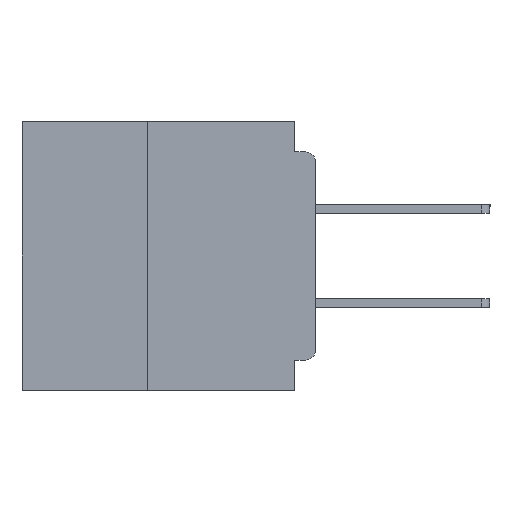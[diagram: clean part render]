
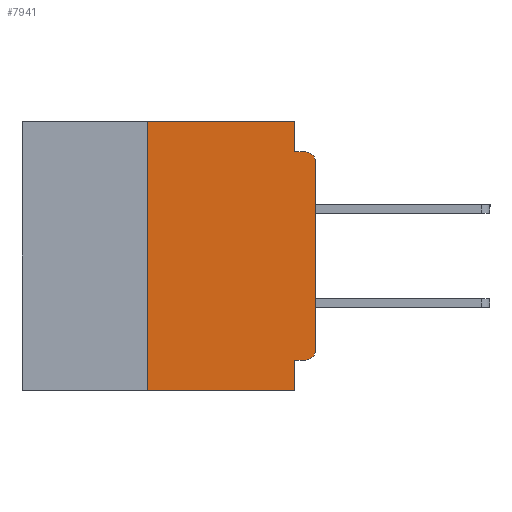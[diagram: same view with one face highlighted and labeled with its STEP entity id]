
A CAD part, left-side view. The second image highlights one B-rep face of the part: STEP entity #7941.
In plain terms, the highlighted planar face has unit normal (-1, 0, 0).
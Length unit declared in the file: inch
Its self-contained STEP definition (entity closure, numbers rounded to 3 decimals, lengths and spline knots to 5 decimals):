
#245 = AXIS2_PLACEMENT_3D ( 'NONE', #40735, #45344, #17824 ) ;
#757 = VERTEX_POINT ( 'NONE', #59119 ) ;
#1016 = CARTESIAN_POINT ( 'NONE',  ( 0., 0.031, -0.4 ) ) ;
#2228 = DIRECTION ( 'NONE',  ( 0., -1., 0. ) ) ;
#2713 = VERTEX_POINT ( 'NONE', #12200 ) ;
#3491 = CARTESIAN_POINT ( 'NONE',  ( 0., 0.25, -0.4 ) ) ;
#3636 = EDGE_CURVE ( 'NONE', #38754, #45544, #35567, .T. ) ;
#3740 = EDGE_CURVE ( 'NONE', #54127, #55398, #32046, .T. ) ;
#5335 = CIRCLE ( 'NONE', #54286, 0.015 ) ;
#5624 = DIRECTION ( 'NONE',  ( 0., 0., 1. ) ) ;
#5644 = DIRECTION ( 'NONE',  ( 0., 0., -1. ) ) ;
#6373 = CARTESIAN_POINT ( 'NONE',  ( 0., 0.437, 0. ) ) ;
#6413 = ORIENTED_EDGE ( 'NONE', *, *, #3740, .F. ) ;
#7406 = VECTOR ( 'NONE', #52155, 39.37008 ) ;
#7941 = ADVANCED_FACE ( 'NONE', ( #8478 ), #8562, .F. ) ;
#8343 = ORIENTED_EDGE ( 'NONE', *, *, #10492, .F. ) ;
#8382 = ORIENTED_EDGE ( 'NONE', *, *, #22914, .F. ) ;
#8478 = FACE_OUTER_BOUND ( 'NONE', #15784, .T. ) ;
#8562 = PLANE ( 'NONE',  #245 ) ;
#8675 = VECTOR ( 'NONE', #56576, 39.37008 ) ;
#8803 = LINE ( 'NONE', #6373, #7406 ) ;
#10492 = EDGE_CURVE ( 'NONE', #46520, #43241, #13922, .T. ) ;
#12200 = CARTESIAN_POINT ( 'NONE',  ( 0., 0.25, 0. ) ) ;
#12949 = LINE ( 'NONE', #29816, #37408 ) ;
#13564 = CARTESIAN_POINT ( 'NONE',  ( 0., 0., -0.34 ) ) ;
#13922 = LINE ( 'NONE', #34553, #35521 ) ;
#14551 = ORIENTED_EDGE ( 'NONE', *, *, #50214, .T. ) ;
#15784 = EDGE_LOOP ( 'NONE', ( #28734, #42595, #8343, #48728, #21454, #20579, #58036, #8382, #6413, #14551 ) ) ;
#17824 = DIRECTION ( 'NONE',  ( 0., 0., -1. ) ) ;
#20398 = CIRCLE ( 'NONE', #53067, 0.015 ) ;
#20579 = ORIENTED_EDGE ( 'NONE', *, *, #39569, .F. ) ;
#20619 = CARTESIAN_POINT ( 'NONE',  ( 0., 0.015, -0.34 ) ) ;
#21454 = ORIENTED_EDGE ( 'NONE', *, *, #31415, .F. ) ;
#22705 = VECTOR ( 'NONE', #30437, 39.37008 ) ;
#22914 = EDGE_CURVE ( 'NONE', #55398, #50740, #23298, .T. ) ;
#23298 = LINE ( 'NONE', #1016, #56996 ) ;
#23340 = VECTOR ( 'NONE', #43967, 39.37008 ) ;
#23410 = CARTESIAN_POINT ( 'NONE',  ( 0., 0., -0.06 ) ) ;
#23478 = LINE ( 'NONE', #33182, #34285 ) ;
#25236 = DIRECTION ( 'NONE',  ( 0., 0., -1. ) ) ;
#27458 = CARTESIAN_POINT ( 'NONE',  ( 0., 0.015, -0.06 ) ) ;
#28734 = ORIENTED_EDGE ( 'NONE', *, *, #3636, .T. ) ;
#29816 = CARTESIAN_POINT ( 'NONE',  ( 0., 0.437, -0.4 ) ) ;
#29907 = VERTEX_POINT ( 'NONE', #3491 ) ;
#30393 = CARTESIAN_POINT ( 'NONE',  ( 0., 0., -0.355 ) ) ;
#30437 = DIRECTION ( 'NONE',  ( 0., 1., 0. ) ) ;
#31415 = EDGE_CURVE ( 'NONE', #2713, #757, #8803, .T. ) ;
#32046 = LINE ( 'NONE', #30393, #22705 ) ;
#32078 = DIRECTION ( 'NONE',  ( 0., 0., -1. ) ) ;
#33182 = CARTESIAN_POINT ( 'NONE',  ( 0., 0.25, -0.4 ) ) ;
#34285 = VECTOR ( 'NONE', #5624, 39.37008 ) ;
#34553 = CARTESIAN_POINT ( 'NONE',  ( 0., 0., -0.045 ) ) ;
#35014 = CARTESIAN_POINT ( 'NONE',  ( 0., 0.015, -0.045 ) ) ;
#35521 = VECTOR ( 'NONE', #39129, 39.37008 ) ;
#35567 = LINE ( 'NONE', #44034, #23340 ) ;
#37261 = CARTESIAN_POINT ( 'NONE',  ( 0., 0.031, -0.045 ) ) ;
#37408 = VECTOR ( 'NONE', #2228, 39.37008 ) ;
#38754 = VERTEX_POINT ( 'NONE', #13564 ) ;
#39129 = DIRECTION ( 'NONE',  ( 0., -1., 0. ) ) ;
#39569 = EDGE_CURVE ( 'NONE', #29907, #2713, #23478, .T. ) ;
#40549 = EDGE_CURVE ( 'NONE', #45544, #43241, #5335, .T. ) ;
#40735 = CARTESIAN_POINT ( 'NONE',  ( 0., 0.437, 0. ) ) ;
#42595 = ORIENTED_EDGE ( 'NONE', *, *, #40549, .T. ) ;
#43241 = VERTEX_POINT ( 'NONE', #35014 ) ;
#43787 = CARTESIAN_POINT ( 'NONE',  ( 0., 0.015, -0.355 ) ) ;
#43953 = EDGE_CURVE ( 'NONE', #29907, #50740, #12949, .T. ) ;
#43967 = DIRECTION ( 'NONE',  ( 0., 0., 1. ) ) ;
#44034 = CARTESIAN_POINT ( 'NONE',  ( 0., 0., 0. ) ) ;
#45344 = DIRECTION ( 'NONE',  ( 1., 0., 0. ) ) ;
#45544 = VERTEX_POINT ( 'NONE', #23410 ) ;
#46325 = EDGE_CURVE ( 'NONE', #757, #46520, #56094, .T. ) ;
#46520 = VERTEX_POINT ( 'NONE', #37261 ) ;
#47054 = CARTESIAN_POINT ( 'NONE',  ( 0., 0.031, -0.4 ) ) ;
#47318 = CARTESIAN_POINT ( 'NONE',  ( 0., 0.031, -0.355 ) ) ;
#48728 = ORIENTED_EDGE ( 'NONE', *, *, #46325, .F. ) ;
#48813 = DIRECTION ( 'NONE',  ( -1., 0., 0. ) ) ;
#50214 = EDGE_CURVE ( 'NONE', #54127, #38754, #20398, .T. ) ;
#50740 = VERTEX_POINT ( 'NONE', #47054 ) ;
#51990 = CARTESIAN_POINT ( 'NONE',  ( 0., 0.031, 0. ) ) ;
#52155 = DIRECTION ( 'NONE',  ( 0., -1., 0. ) ) ;
#52724 = DIRECTION ( 'NONE',  ( -1., 0., 0. ) ) ;
#53067 = AXIS2_PLACEMENT_3D ( 'NONE', #20619, #52724, #25236 ) ;
#54127 = VERTEX_POINT ( 'NONE', #43787 ) ;
#54286 = AXIS2_PLACEMENT_3D ( 'NONE', #27458, #48813, #32078 ) ;
#55398 = VERTEX_POINT ( 'NONE', #47318 ) ;
#56094 = LINE ( 'NONE', #51990, #8675 ) ;
#56576 = DIRECTION ( 'NONE',  ( 0., 0., -1. ) ) ;
#56996 = VECTOR ( 'NONE', #5644, 39.37008 ) ;
#58036 = ORIENTED_EDGE ( 'NONE', *, *, #43953, .T. ) ;
#59119 = CARTESIAN_POINT ( 'NONE',  ( 0., 0.031, 0. ) ) ;
